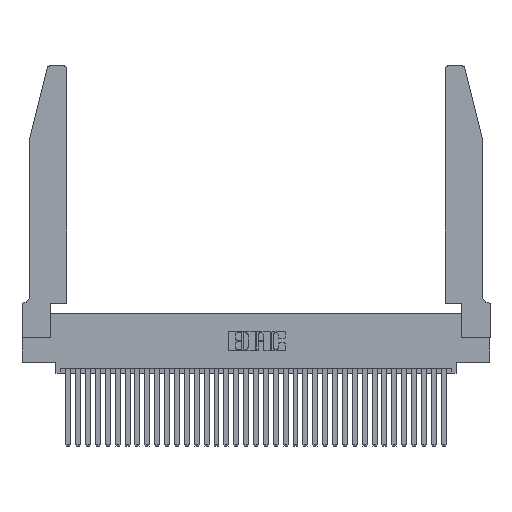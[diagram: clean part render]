
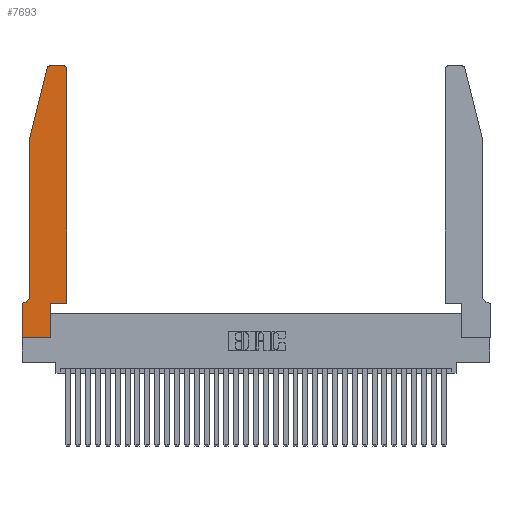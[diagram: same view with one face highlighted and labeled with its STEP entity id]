
A CAD part, top view. The second image highlights one B-rep face of the part: STEP entity #7693.
In plain terms, the highlighted planar face has unit normal (0, 0, 1).
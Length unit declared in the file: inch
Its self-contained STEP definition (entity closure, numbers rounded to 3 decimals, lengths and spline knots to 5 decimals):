
#17 = VECTOR ( 'NONE', #28442, 39.37008 ) ;
#477 = EDGE_CURVE ( 'NONE', #28360, #18851, #13348, .T. ) ;
#1110 = DIRECTION ( 'NONE',  ( 0., -1., 0. ) ) ;
#1334 = ORIENTED_EDGE ( 'NONE', *, *, #7035, .T. ) ;
#1441 = VERTEX_POINT ( 'NONE', #31599 ) ;
#1610 = DIRECTION ( 'NONE',  ( 0., 0., 1. ) ) ;
#1992 = CARTESIAN_POINT ( 'NONE',  ( 0.284, 2.72, 0.37 ) ) ;
#1995 = DIRECTION ( 'NONE',  ( 1., 0., 0. ) ) ;
#2029 = CARTESIAN_POINT ( 'NONE',  ( 0.2865, 0.35, 0.37 ) ) ;
#2244 = CARTESIAN_POINT ( 'NONE',  ( 0., 0., 0.37 ) ) ;
#3278 = VECTOR ( 'NONE', #29651, 39.37008 ) ;
#3698 = LINE ( 'NONE', #23307, #32164 ) ;
#3987 = FACE_OUTER_BOUND ( 'NONE', #20285, .T. ) ;
#4009 = EDGE_CURVE ( 'NONE', #13819, #21435, #22218, .T. ) ;
#4111 = EDGE_CURVE ( 'NONE', #14086, #13819, #20510, .T. ) ;
#4367 = LINE ( 'NONE', #14277, #18294 ) ;
#4808 = DIRECTION ( 'NONE',  ( 1., 0., 0. ) ) ;
#6716 = CARTESIAN_POINT ( 'NONE',  ( 0.0055, 0.35, 0.37 ) ) ;
#7035 = EDGE_CURVE ( 'NONE', #21435, #1441, #31188, .T. ) ;
#7538 = VECTOR ( 'NONE', #10061, 39.37008 ) ;
#7693 = ADVANCED_FACE ( 'NONE', ( #3987 ), #31890, .T. ) ;
#8415 = VECTOR ( 'NONE', #19187, 39.37008 ) ;
#8944 = EDGE_CURVE ( 'NONE', #18851, #9084, #30657, .T. ) ;
#8954 = CARTESIAN_POINT ( 'NONE',  ( 0., 0.35, 0.37 ) ) ;
#9084 = VERTEX_POINT ( 'NONE', #27326 ) ;
#9836 = CIRCLE ( 'NONE', #35589, 0.07 ) ;
#9946 = CARTESIAN_POINT ( 'NONE',  ( 0.4505, 0.35, 0.37 ) ) ;
#10061 = DIRECTION ( 'NONE',  ( 1., 0., 0. ) ) ;
#10391 = DIRECTION ( 'NONE',  ( 0., -1., 0. ) ) ;
#10806 = CARTESIAN_POINT ( 'NONE',  ( 0.4505, 2.72, 0.37 ) ) ;
#10951 = ORIENTED_EDGE ( 'NONE', *, *, #14867, .T. ) ;
#13348 = LINE ( 'NONE', #2244, #34370 ) ;
#13369 = CARTESIAN_POINT ( 'NONE',  ( 0.4505, 0.35, 0.37 ) ) ;
#13748 = ORIENTED_EDGE ( 'NONE', *, *, #31050, .T. ) ;
#13819 = VERTEX_POINT ( 'NONE', #26097 ) ;
#14076 = CARTESIAN_POINT ( 'NONE',  ( 0.0055, 0.42, 0.37 ) ) ;
#14086 = VERTEX_POINT ( 'NONE', #10806 ) ;
#14277 = CARTESIAN_POINT ( 'NONE',  ( 0.0755, 2., 0.37 ) ) ;
#14316 = AXIS2_PLACEMENT_3D ( 'NONE', #1992, #21406, #4808 ) ;
#14867 = EDGE_CURVE ( 'NONE', #25105, #28360, #29374, .T. ) ;
#14969 = LINE ( 'NONE', #35501, #8415 ) ;
#15159 = CARTESIAN_POINT ( 'NONE',  ( 0.0755, 0.42, 0.37 ) ) ;
#15178 = VERTEX_POINT ( 'NONE', #23992 ) ;
#16872 = DIRECTION ( 'NONE',  ( -1., 0., 0. ) ) ;
#17070 = DIRECTION ( 'NONE',  ( -0.239, -0.971, 0. ) ) ;
#17080 = EDGE_CURVE ( 'NONE', #34959, #25105, #9836, .T. ) ;
#18280 = CARTESIAN_POINT ( 'NONE',  ( 0., 0.35, 0.37 ) ) ;
#18294 = VECTOR ( 'NONE', #17070, 39.37008 ) ;
#18851 = VERTEX_POINT ( 'NONE', #19077 ) ;
#19077 = CARTESIAN_POINT ( 'NONE',  ( 0., 0., 0.37 ) ) ;
#19187 = DIRECTION ( 'NONE',  ( 0., 1., 0. ) ) ;
#19254 = CARTESIAN_POINT ( 'NONE',  ( 0.284, 2.75, 0.37 ) ) ;
#20285 = EDGE_LOOP ( 'NONE', ( #24430, #1334, #28088, #32177, #33117, #10951, #30216, #34451, #21966, #24137, #13748, #30435 ) ) ;
#20322 = CARTESIAN_POINT ( 'NONE',  ( 0.2865, 0.35, 0.37 ) ) ;
#20365 = AXIS2_PLACEMENT_3D ( 'NONE', #18280, #1610, #21026 ) ;
#20510 = CIRCLE ( 'NONE', #29183, 0.03 ) ;
#21026 = DIRECTION ( 'NONE',  ( 1., 0., 0. ) ) ;
#21274 = VECTOR ( 'NONE', #33675, 39.37008 ) ;
#21406 = DIRECTION ( 'NONE',  ( 0., 0., 1. ) ) ;
#21410 = CARTESIAN_POINT ( 'NONE',  ( 0., 0., 0.37 ) ) ;
#21435 = VERTEX_POINT ( 'NONE', #19254 ) ;
#21966 = ORIENTED_EDGE ( 'NONE', *, *, #33306, .T. ) ;
#22143 = EDGE_CURVE ( 'NONE', #1441, #15178, #4367, .T. ) ;
#22218 = LINE ( 'NONE', #33835, #17 ) ;
#23307 = CARTESIAN_POINT ( 'NONE',  ( 0.0755, 2., 0.37 ) ) ;
#23447 = VECTOR ( 'NONE', #1995, 39.37008 ) ;
#23992 = CARTESIAN_POINT ( 'NONE',  ( 0.0755, 2., 0.37 ) ) ;
#24137 = ORIENTED_EDGE ( 'NONE', *, *, #31531, .T. ) ;
#24430 = ORIENTED_EDGE ( 'NONE', *, *, #4009, .T. ) ;
#25101 = EDGE_CURVE ( 'NONE', #15178, #34959, #3698, .T. ) ;
#25105 = VERTEX_POINT ( 'NONE', #6716 ) ;
#25326 = LINE ( 'NONE', #2029, #3278 ) ;
#26097 = CARTESIAN_POINT ( 'NONE',  ( 0.4205, 2.75, 0.37 ) ) ;
#27326 = CARTESIAN_POINT ( 'NONE',  ( 0.2865, 0., 0.37 ) ) ;
#28088 = ORIENTED_EDGE ( 'NONE', *, *, #22143, .T. ) ;
#28360 = VERTEX_POINT ( 'NONE', #8954 ) ;
#28442 = DIRECTION ( 'NONE',  ( -1., 0., 0. ) ) ;
#28628 = CARTESIAN_POINT ( 'NONE',  ( 0.4205, 2.72, 0.37 ) ) ;
#29183 = AXIS2_PLACEMENT_3D ( 'NONE', #28628, #32689, #30733 ) ;
#29374 = LINE ( 'NONE', #30790, #21274 ) ;
#29651 = DIRECTION ( 'NONE',  ( 0., 1., 0. ) ) ;
#30216 = ORIENTED_EDGE ( 'NONE', *, *, #477, .T. ) ;
#30336 = LINE ( 'NONE', #9946, #7538 ) ;
#30435 = ORIENTED_EDGE ( 'NONE', *, *, #4111, .T. ) ;
#30657 = LINE ( 'NONE', #21410, #23447 ) ;
#30733 = DIRECTION ( 'NONE',  ( 1., 0., 0. ) ) ;
#30790 = CARTESIAN_POINT ( 'NONE',  ( 0.0755, 0.35, 0.37 ) ) ;
#31008 = VERTEX_POINT ( 'NONE', #13369 ) ;
#31050 = EDGE_CURVE ( 'NONE', #31008, #14086, #14969, .T. ) ;
#31188 = CIRCLE ( 'NONE', #14316, 0.03 ) ;
#31531 = EDGE_CURVE ( 'NONE', #31973, #31008, #30336, .T. ) ;
#31599 = CARTESIAN_POINT ( 'NONE',  ( 0.25487, 2.72718, 0.37 ) ) ;
#31890 = PLANE ( 'NONE',  #20365 ) ;
#31973 = VERTEX_POINT ( 'NONE', #20322 ) ;
#32164 = VECTOR ( 'NONE', #1110, 39.37008 ) ;
#32177 = ORIENTED_EDGE ( 'NONE', *, *, #25101, .T. ) ;
#32689 = DIRECTION ( 'NONE',  ( 0., 0., 1. ) ) ;
#33117 = ORIENTED_EDGE ( 'NONE', *, *, #17080, .T. ) ;
#33243 = DIRECTION ( 'NONE',  ( 0., 0., -1. ) ) ;
#33306 = EDGE_CURVE ( 'NONE', #9084, #31973, #25326, .T. ) ;
#33675 = DIRECTION ( 'NONE',  ( -1., 0., 0. ) ) ;
#33835 = CARTESIAN_POINT ( 'NONE',  ( 0.2605, 2.75, 0.37 ) ) ;
#34370 = VECTOR ( 'NONE', #10391, 39.37008 ) ;
#34451 = ORIENTED_EDGE ( 'NONE', *, *, #8944, .T. ) ;
#34959 = VERTEX_POINT ( 'NONE', #15159 ) ;
#35501 = CARTESIAN_POINT ( 'NONE',  ( 0.4505, 0.35, 0.37 ) ) ;
#35589 = AXIS2_PLACEMENT_3D ( 'NONE', #14076, #33243, #16872 ) ;
